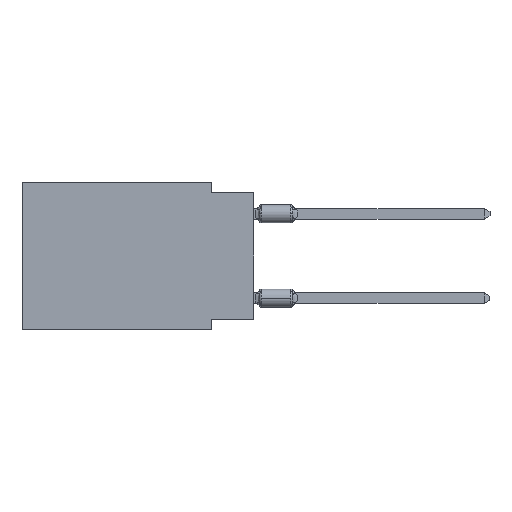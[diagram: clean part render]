
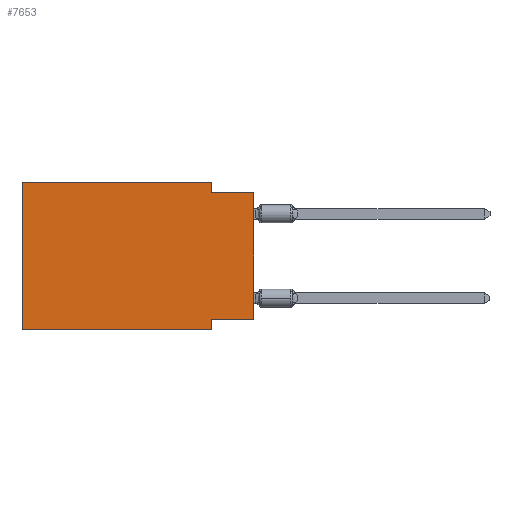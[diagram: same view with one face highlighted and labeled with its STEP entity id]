
A CAD part, left-side view. The second image highlights one B-rep face of the part: STEP entity #7653.
In plain terms, the highlighted planar face has unit normal (-1, 0, 0).
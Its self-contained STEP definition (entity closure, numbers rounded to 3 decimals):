
#196 = CARTESIAN_POINT ( 'NONE',  ( 0., 0., -8.255 ) ) ;
#213 = VERTEX_POINT ( 'NONE', #11107 ) ;
#1200 = CARTESIAN_POINT ( 'NONE',  ( 0., 13.97, -8.89 ) ) ;
#1806 = EDGE_LOOP ( 'NONE', ( #13087, #4848, #6976, #9999, #7169, #4148, #3117, #2947 ) ) ;
#1857 = LINE ( 'NONE', #9903, #6713 ) ;
#1866 = EDGE_CURVE ( 'NONE', #6513, #5339, #8230, .T. ) ;
#2079 = DIRECTION ( 'NONE',  ( 1., 0., 0. ) ) ;
#2682 = VERTEX_POINT ( 'NONE', #4288 ) ;
#2783 = DIRECTION ( 'NONE',  ( 0., 0., -1. ) ) ;
#2947 = ORIENTED_EDGE ( 'NONE', *, *, #5953, .F. ) ;
#3052 = DIRECTION ( 'NONE',  ( 0., -1., 0. ) ) ;
#3117 = ORIENTED_EDGE ( 'NONE', *, *, #9841, .F. ) ;
#3196 = VECTOR ( 'NONE', #10276, 1000. ) ;
#3575 = CARTESIAN_POINT ( 'NONE',  ( 0., 13.97, 0. ) ) ;
#3678 = VECTOR ( 'NONE', #2783, 1000. ) ;
#3793 = CARTESIAN_POINT ( 'NONE',  ( 0., 0., -0.635 ) ) ;
#3794 = CARTESIAN_POINT ( 'NONE',  ( 0., 2.54, -8.89 ) ) ;
#4134 = DIRECTION ( 'NONE',  ( 0., 0., -1. ) ) ;
#4148 = ORIENTED_EDGE ( 'NONE', *, *, #6548, .T. ) ;
#4190 = VECTOR ( 'NONE', #4134, 1000. ) ;
#4247 = DIRECTION ( 'NONE',  ( 0., -1., 0. ) ) ;
#4288 = CARTESIAN_POINT ( 'NONE',  ( 0., 2.54, -8.89 ) ) ;
#4526 = VERTEX_POINT ( 'NONE', #12191 ) ;
#4652 = VERTEX_POINT ( 'NONE', #196 ) ;
#4821 = LINE ( 'NONE', #3794, #3678 ) ;
#4848 = ORIENTED_EDGE ( 'NONE', *, *, #10274, .F. ) ;
#4999 = VECTOR ( 'NONE', #3052, 1000. ) ;
#5145 = FACE_OUTER_BOUND ( 'NONE', #1806, .T. ) ;
#5339 = VERTEX_POINT ( 'NONE', #9398 ) ;
#5830 = EDGE_CURVE ( 'NONE', #213, #10620, #13414, .T. ) ;
#5953 = EDGE_CURVE ( 'NONE', #4652, #4526, #10680, .T. ) ;
#6116 = LINE ( 'NONE', #8367, #3196 ) ;
#6186 = DIRECTION ( 'NONE',  ( 0., 0., 1. ) ) ;
#6217 = VECTOR ( 'NONE', #6186, 1000. ) ;
#6231 = PLANE ( 'NONE',  #8861 ) ;
#6513 = VERTEX_POINT ( 'NONE', #12706 ) ;
#6548 = EDGE_CURVE ( 'NONE', #213, #2682, #11624, .T. ) ;
#6713 = VECTOR ( 'NONE', #11960, 1000. ) ;
#6746 = CARTESIAN_POINT ( 'NONE',  ( 0., 0., -0.635 ) ) ;
#6976 = ORIENTED_EDGE ( 'NONE', *, *, #1866, .F. ) ;
#7169 = ORIENTED_EDGE ( 'NONE', *, *, #5830, .F. ) ;
#7213 = CARTESIAN_POINT ( 'NONE',  ( 0., 13.97, 0. ) ) ;
#7259 = EDGE_CURVE ( 'NONE', #4652, #13236, #6116, .T. ) ;
#7653 = ADVANCED_FACE ( 'NONE', ( #5145 ), #6231, .F. ) ;
#8230 = LINE ( 'NONE', #8301, #4190 ) ;
#8301 = CARTESIAN_POINT ( 'NONE',  ( 0., 2.54, 0. ) ) ;
#8367 = CARTESIAN_POINT ( 'NONE',  ( 0., 0., 0. ) ) ;
#8635 = CARTESIAN_POINT ( 'NONE',  ( 0., 0., -8.255 ) ) ;
#8861 = AXIS2_PLACEMENT_3D ( 'NONE', #13326, #2079, #10466 ) ;
#9072 = EDGE_CURVE ( 'NONE', #10620, #6513, #1857, .T. ) ;
#9398 = CARTESIAN_POINT ( 'NONE',  ( 0., 2.54, -0.635 ) ) ;
#9841 = EDGE_CURVE ( 'NONE', #4526, #2682, #4821, .T. ) ;
#9903 = CARTESIAN_POINT ( 'NONE',  ( 0., 13.97, 0. ) ) ;
#9999 = ORIENTED_EDGE ( 'NONE', *, *, #9072, .F. ) ;
#10274 = EDGE_CURVE ( 'NONE', #5339, #13236, #12125, .T. ) ;
#10276 = DIRECTION ( 'NONE',  ( 0., 0., 1. ) ) ;
#10466 = DIRECTION ( 'NONE',  ( 0., 0., -1. ) ) ;
#10620 = VERTEX_POINT ( 'NONE', #3575 ) ;
#10680 = LINE ( 'NONE', #8635, #11882 ) ;
#11107 = CARTESIAN_POINT ( 'NONE',  ( 0., 13.97, -8.89 ) ) ;
#11244 = VECTOR ( 'NONE', #4247, 1000. ) ;
#11624 = LINE ( 'NONE', #1200, #11244 ) ;
#11882 = VECTOR ( 'NONE', #12794, 1000. ) ;
#11960 = DIRECTION ( 'NONE',  ( 0., -1., 0. ) ) ;
#12125 = LINE ( 'NONE', #3793, #4999 ) ;
#12191 = CARTESIAN_POINT ( 'NONE',  ( 0., 2.54, -8.255 ) ) ;
#12706 = CARTESIAN_POINT ( 'NONE',  ( 0., 2.54, 0. ) ) ;
#12794 = DIRECTION ( 'NONE',  ( 0., 1., 0. ) ) ;
#13087 = ORIENTED_EDGE ( 'NONE', *, *, #7259, .T. ) ;
#13236 = VERTEX_POINT ( 'NONE', #6746 ) ;
#13326 = CARTESIAN_POINT ( 'NONE',  ( 0., 13.97, 0. ) ) ;
#13414 = LINE ( 'NONE', #7213, #6217 ) ;
